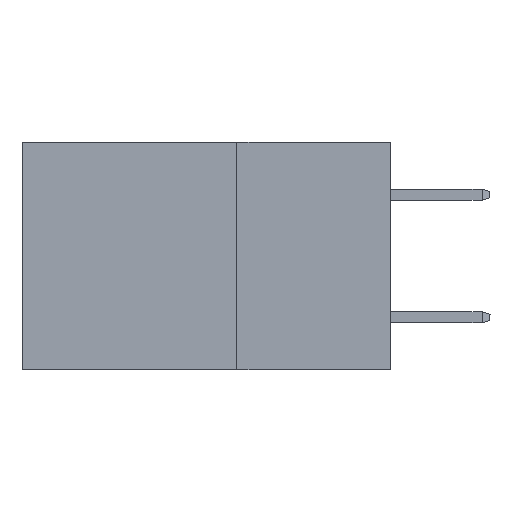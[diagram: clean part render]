
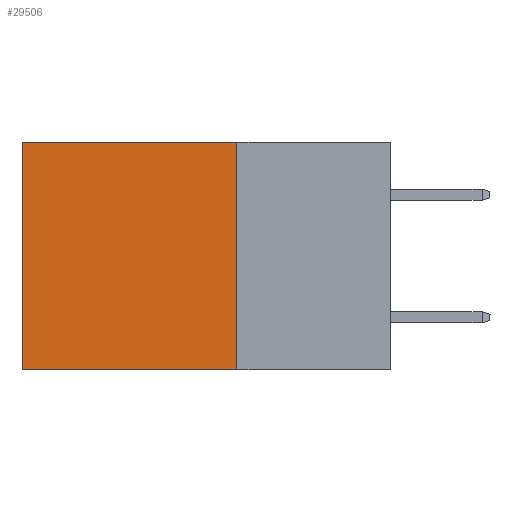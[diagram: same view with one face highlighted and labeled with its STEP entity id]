
A CAD part, left-side view. The second image highlights one B-rep face of the part: STEP entity #29506.
In plain terms, the highlighted planar face has unit normal (-1, 0, 0).
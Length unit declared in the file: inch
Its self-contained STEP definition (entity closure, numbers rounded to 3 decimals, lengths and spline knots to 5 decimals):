
#463 = DIRECTION ( 'NONE',  ( 0., 0., -1. ) ) ;
#5334 = VECTOR ( 'NONE', #26119, 39.37008 ) ;
#6229 = ORIENTED_EDGE ( 'NONE', *, *, #27201, .F. ) ;
#6745 = DIRECTION ( 'NONE',  ( 0., 1., 0. ) ) ;
#6788 = VECTOR ( 'NONE', #12133, 39.37008 ) ;
#6793 = DIRECTION ( 'NONE',  ( 1., 0., 0. ) ) ;
#8377 = CARTESIAN_POINT ( 'NONE',  ( 0.2875, 0.25, 0. ) ) ;
#9255 = ORIENTED_EDGE ( 'NONE', *, *, #17873, .T. ) ;
#9702 = VERTEX_POINT ( 'NONE', #24600 ) ;
#10273 = CARTESIAN_POINT ( 'NONE',  ( 0.2875, 0.25, 0. ) ) ;
#10391 = VERTEX_POINT ( 'NONE', #28581 ) ;
#11801 = LINE ( 'NONE', #8377, #26543 ) ;
#12133 = DIRECTION ( 'NONE',  ( 0., 0., -1. ) ) ;
#15524 = VECTOR ( 'NONE', #6745, 39.37008 ) ;
#15601 = EDGE_CURVE ( 'NONE', #9702, #10391, #25574, .T. ) ;
#17873 = EDGE_CURVE ( 'NONE', #26804, #9702, #41008, .T. ) ;
#19913 = PLANE ( 'NONE',  #33358 ) ;
#23545 = ORIENTED_EDGE ( 'NONE', *, *, #38801, .F. ) ;
#24560 = VERTEX_POINT ( 'NONE', #33333 ) ;
#24600 = CARTESIAN_POINT ( 'NONE',  ( 0.2875, 0.6, 0. ) ) ;
#25346 = CARTESIAN_POINT ( 'NONE',  ( 0.2875, 0.6, 0. ) ) ;
#25574 = LINE ( 'NONE', #25346, #6788 ) ;
#26119 = DIRECTION ( 'NONE',  ( 0., 1., 0. ) ) ;
#26170 = ORIENTED_EDGE ( 'NONE', *, *, #15601, .T. ) ;
#26543 = VECTOR ( 'NONE', #27535, 39.37008 ) ;
#26804 = VERTEX_POINT ( 'NONE', #27720 ) ;
#27201 = EDGE_CURVE ( 'NONE', #24560, #10391, #29727, .T. ) ;
#27354 = EDGE_LOOP ( 'NONE', ( #26170, #6229, #23545, #9255 ) ) ;
#27535 = DIRECTION ( 'NONE',  ( 0., 0., -1. ) ) ;
#27720 = CARTESIAN_POINT ( 'NONE',  ( 0.2875, 0.25, 0. ) ) ;
#28581 = CARTESIAN_POINT ( 'NONE',  ( 0.2875, 0.6, -0.37 ) ) ;
#29506 = ADVANCED_FACE ( 'NONE', ( #29553 ), #19913, .F. ) ;
#29553 = FACE_OUTER_BOUND ( 'NONE', #27354, .T. ) ;
#29727 = LINE ( 'NONE', #35796, #5334 ) ;
#33333 = CARTESIAN_POINT ( 'NONE',  ( 0.2875, 0.25, -0.37 ) ) ;
#33358 = AXIS2_PLACEMENT_3D ( 'NONE', #39320, #6793, #463 ) ;
#35796 = CARTESIAN_POINT ( 'NONE',  ( 0.2875, 0.25, -0.37 ) ) ;
#38801 = EDGE_CURVE ( 'NONE', #26804, #24560, #11801, .T. ) ;
#39320 = CARTESIAN_POINT ( 'NONE',  ( 0.2875, 0.25, 0. ) ) ;
#41008 = LINE ( 'NONE', #10273, #15524 ) ;
